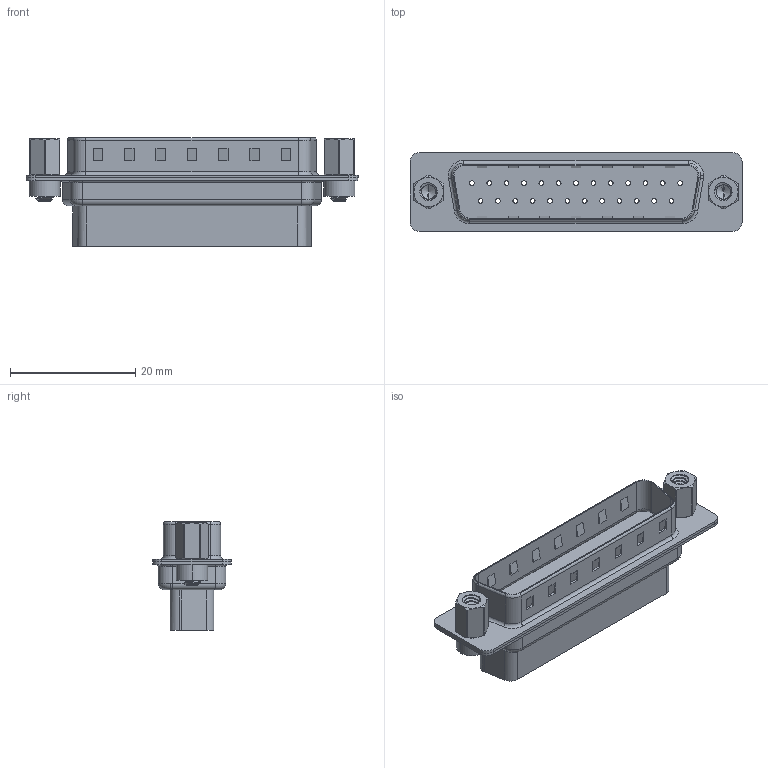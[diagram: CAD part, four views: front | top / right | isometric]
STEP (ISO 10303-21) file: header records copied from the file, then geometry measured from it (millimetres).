
FILE_DESCRIPTION (( 'STEP AP203' ), '1' );
FILE_NAME ('627-025-010-043.STEP', '2020-07-15T20:36:02', ( '' ), ( '' ), 'SwSTEP 2.0', 'SolidWorks 2020', '' );
FILE_SCHEMA (( 'CONFIG_CONTROL_DESIGN' ));
Length unit declared in the file: millimetre
Products named in the file (6): 627 Shell Front_25 Contacts; 627-025-010-043; 627 Shell Rear_25 Contacts; 627 Housing_25 HP; 627 4-40 Threaded Rivet; 627 4-40 Hex Standoff
Assembly tree (7 placements, depth 2):
  627-025-010-043
    627 Housing_25 HP
    627 Shell Front_25 Contacts
    627 Shell Rear_25 Contacts
    627 4-40 Threaded Rivet  x2
    627 4-40 Hex Standoff  x2
Bounding box: 53 x 12.6 x 17.4 mm (x, y, z)
Volume: 3713.2 mm3; surface area: 7091 mm2
Topology: 7 solids, 7 shells, 698 faces, 1745 edges, 1122 vertices
Faces by surface type: cylinder 357, plane 243, torus 50, cone 30, bspline 18
Entity records: 22876 total; most frequent: CARTESIAN_POINT 7472, DIRECTION 3185, ORIENTED_EDGE 2986, EDGE_CURVE 1493, AXIS2_PLACEMENT_3D 1223, VERTEX_POINT 960, EDGE_LOOP 757, VECTOR 739
